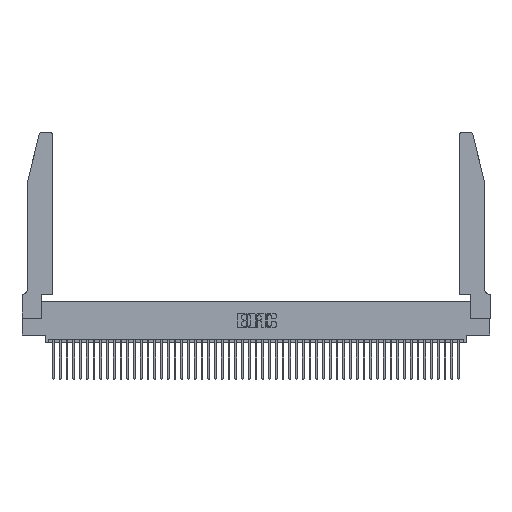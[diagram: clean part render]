
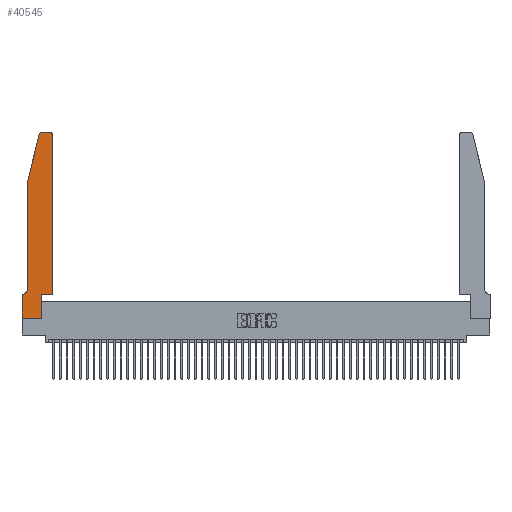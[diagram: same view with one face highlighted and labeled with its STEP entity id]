
A CAD part, top view. The second image highlights one B-rep face of the part: STEP entity #40545.
In plain terms, the highlighted planar face has unit normal (0, 0, 1).
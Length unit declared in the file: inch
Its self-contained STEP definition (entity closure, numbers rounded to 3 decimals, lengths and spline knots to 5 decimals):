
#895 = AXIS2_PLACEMENT_3D ( 'NONE', #5784, #1733, #40382 ) ;
#1687 = ORIENTED_EDGE ( 'NONE', *, *, #38924, .T. ) ;
#1733 = DIRECTION ( 'NONE',  ( 0., 0., 1. ) ) ;
#1961 = AXIS2_PLACEMENT_3D ( 'NONE', #10646, #10140, #18098 ) ;
#3257 = CARTESIAN_POINT ( 'NONE',  ( 0.2605, 2.75, 0.37 ) ) ;
#4375 = ORIENTED_EDGE ( 'NONE', *, *, #48775, .T. ) ;
#4608 = LINE ( 'NONE', #48149, #23422 ) ;
#4831 = EDGE_CURVE ( 'NONE', #44853, #16241, #30279, .T. ) ;
#4845 = ORIENTED_EDGE ( 'NONE', *, *, #49633, .T. ) ;
#5235 = EDGE_CURVE ( 'NONE', #25464, #12131, #12644, .T. ) ;
#5326 = VERTEX_POINT ( 'NONE', #26094 ) ;
#5435 = CARTESIAN_POINT ( 'NONE',  ( 0.4505, 0.35, 0.37 ) ) ;
#5784 = CARTESIAN_POINT ( 'NONE',  ( 0.284, 2.72, 0.37 ) ) ;
#5933 = CARTESIAN_POINT ( 'NONE',  ( 0.0755, 2., 0.37 ) ) ;
#7418 = EDGE_CURVE ( 'NONE', #37153, #15062, #4608, .T. ) ;
#8708 = PLANE ( 'NONE',  #10379 ) ;
#8995 = CARTESIAN_POINT ( 'NONE',  ( 0.2865, 0.35, 0.37 ) ) ;
#9903 = EDGE_CURVE ( 'NONE', #29496, #5326, #27393, .T. ) ;
#10049 = EDGE_CURVE ( 'NONE', #49851, #44853, #29752, .T. ) ;
#10064 = VECTOR ( 'NONE', #48953, 39.37008 ) ;
#10140 = DIRECTION ( 'NONE',  ( 0., 0., -1. ) ) ;
#10379 = AXIS2_PLACEMENT_3D ( 'NONE', #28350, #28513, #24805 ) ;
#10646 = CARTESIAN_POINT ( 'NONE',  ( 0.0055, 0.42, 0.37 ) ) ;
#10934 = CARTESIAN_POINT ( 'NONE',  ( 0.2865, 0., 0.37 ) ) ;
#11265 = CARTESIAN_POINT ( 'NONE',  ( 0.25487, 2.72718, 0.37 ) ) ;
#11903 = DIRECTION ( 'NONE',  ( 0., -1., 0. ) ) ;
#12131 = VERTEX_POINT ( 'NONE', #30305 ) ;
#12159 = DIRECTION ( 'NONE',  ( 0., 0., 1. ) ) ;
#12335 = VERTEX_POINT ( 'NONE', #20091 ) ;
#12644 = LINE ( 'NONE', #22041, #34484 ) ;
#12860 = DIRECTION ( 'NONE',  ( 0., -1., 0. ) ) ;
#15062 = VERTEX_POINT ( 'NONE', #40187 ) ;
#15099 = CARTESIAN_POINT ( 'NONE',  ( 0.4505, 0.35, 0.37 ) ) ;
#15204 = EDGE_CURVE ( 'NONE', #5326, #25464, #15318, .T. ) ;
#15313 = EDGE_CURVE ( 'NONE', #16241, #20858, #47471, .T. ) ;
#15318 = LINE ( 'NONE', #5435, #43827 ) ;
#16241 = VERTEX_POINT ( 'NONE', #36852 ) ;
#16560 = FACE_OUTER_BOUND ( 'NONE', #43629, .T. ) ;
#16762 = LINE ( 'NONE', #29061, #10064 ) ;
#17119 = VECTOR ( 'NONE', #35952, 39.37008 ) ;
#18098 = DIRECTION ( 'NONE',  ( -1., 0., 0. ) ) ;
#18165 = VECTOR ( 'NONE', #26978, 39.37008 ) ;
#20091 = CARTESIAN_POINT ( 'NONE',  ( 0.284, 2.75, 0.37 ) ) ;
#20858 = VERTEX_POINT ( 'NONE', #25593 ) ;
#22041 = CARTESIAN_POINT ( 'NONE',  ( 0.4505, 0.35, 0.37 ) ) ;
#23422 = VECTOR ( 'NONE', #12860, 39.37008 ) ;
#23681 = ORIENTED_EDGE ( 'NONE', *, *, #46556, .T. ) ;
#24133 = CIRCLE ( 'NONE', #895, 0.03 ) ;
#24805 = DIRECTION ( 'NONE',  ( 1., 0., 0. ) ) ;
#25464 = VERTEX_POINT ( 'NONE', #15099 ) ;
#25593 = CARTESIAN_POINT ( 'NONE',  ( 0.0055, 0.35, 0.37 ) ) ;
#25927 = DIRECTION ( 'NONE',  ( 0., 1., 0. ) ) ;
#26094 = CARTESIAN_POINT ( 'NONE',  ( 0.2865, 0.35, 0.37 ) ) ;
#26978 = DIRECTION ( 'NONE',  ( -1., 0., 0. ) ) ;
#27210 = EDGE_CURVE ( 'NONE', #30977, #12335, #43808, .T. ) ;
#27241 = AXIS2_PLACEMENT_3D ( 'NONE', #35045, #12159, #39313 ) ;
#27393 = LINE ( 'NONE', #8995, #17119 ) ;
#28350 = CARTESIAN_POINT ( 'NONE',  ( 0., 0.35, 0.37 ) ) ;
#28431 = VECTOR ( 'NONE', #11903, 39.37008 ) ;
#28513 = DIRECTION ( 'NONE',  ( 0., 0., 1. ) ) ;
#28637 = VECTOR ( 'NONE', #42072, 39.37008 ) ;
#29061 = CARTESIAN_POINT ( 'NONE',  ( 0., 0., 0.37 ) ) ;
#29496 = VERTEX_POINT ( 'NONE', #10934 ) ;
#29752 = LINE ( 'NONE', #32724, #48016 ) ;
#30279 = LINE ( 'NONE', #42800, #28431 ) ;
#30305 = CARTESIAN_POINT ( 'NONE',  ( 0.4505, 2.72, 0.37 ) ) ;
#30977 = VERTEX_POINT ( 'NONE', #37005 ) ;
#31026 = ORIENTED_EDGE ( 'NONE', *, *, #9903, .T. ) ;
#32724 = CARTESIAN_POINT ( 'NONE',  ( 0.0755, 2., 0.37 ) ) ;
#33470 = ORIENTED_EDGE ( 'NONE', *, *, #5235, .T. ) ;
#34265 = ORIENTED_EDGE ( 'NONE', *, *, #15313, .T. ) ;
#34484 = VECTOR ( 'NONE', #25927, 39.37008 ) ;
#34774 = CARTESIAN_POINT ( 'NONE',  ( 0.0755, 0.35, 0.37 ) ) ;
#34918 = CIRCLE ( 'NONE', #27241, 0.03 ) ;
#35045 = CARTESIAN_POINT ( 'NONE',  ( 0.4205, 2.72, 0.37 ) ) ;
#35952 = DIRECTION ( 'NONE',  ( 0., 1., 0. ) ) ;
#36774 = DIRECTION ( 'NONE',  ( -0.239, -0.971, 0. ) ) ;
#36852 = CARTESIAN_POINT ( 'NONE',  ( 0.0755, 0.42, 0.37 ) ) ;
#37005 = CARTESIAN_POINT ( 'NONE',  ( 0.4205, 2.75, 0.37 ) ) ;
#37153 = VERTEX_POINT ( 'NONE', #43700 ) ;
#38924 = EDGE_CURVE ( 'NONE', #12131, #30977, #34918, .T. ) ;
#39313 = DIRECTION ( 'NONE',  ( 1., 0., 0. ) ) ;
#40062 = ORIENTED_EDGE ( 'NONE', *, *, #4831, .T. ) ;
#40187 = CARTESIAN_POINT ( 'NONE',  ( 0., 0., 0.37 ) ) ;
#40353 = DIRECTION ( 'NONE',  ( 1., 0., 0. ) ) ;
#40382 = DIRECTION ( 'NONE',  ( 1., 0., 0. ) ) ;
#40545 = ADVANCED_FACE ( 'NONE', ( #16560 ), #8708, .T. ) ;
#41260 = ORIENTED_EDGE ( 'NONE', *, *, #27210, .T. ) ;
#41437 = ORIENTED_EDGE ( 'NONE', *, *, #10049, .T. ) ;
#42072 = DIRECTION ( 'NONE',  ( -1., 0., 0. ) ) ;
#42800 = CARTESIAN_POINT ( 'NONE',  ( 0.0755, 2., 0.37 ) ) ;
#42961 = ORIENTED_EDGE ( 'NONE', *, *, #7418, .T. ) ;
#43629 = EDGE_LOOP ( 'NONE', ( #41260, #4375, #41437, #40062, #34265, #23681, #42961, #4845, #31026, #48952, #33470, #1687 ) ) ;
#43700 = CARTESIAN_POINT ( 'NONE',  ( 0., 0.35, 0.37 ) ) ;
#43808 = LINE ( 'NONE', #3257, #28637 ) ;
#43827 = VECTOR ( 'NONE', #40353, 39.37008 ) ;
#44853 = VERTEX_POINT ( 'NONE', #5933 ) ;
#46556 = EDGE_CURVE ( 'NONE', #20858, #37153, #47340, .T. ) ;
#47340 = LINE ( 'NONE', #34774, #18165 ) ;
#47471 = CIRCLE ( 'NONE', #1961, 0.07 ) ;
#48016 = VECTOR ( 'NONE', #36774, 39.37008 ) ;
#48149 = CARTESIAN_POINT ( 'NONE',  ( 0., 0., 0.37 ) ) ;
#48775 = EDGE_CURVE ( 'NONE', #12335, #49851, #24133, .T. ) ;
#48952 = ORIENTED_EDGE ( 'NONE', *, *, #15204, .T. ) ;
#48953 = DIRECTION ( 'NONE',  ( 1., 0., 0. ) ) ;
#49633 = EDGE_CURVE ( 'NONE', #15062, #29496, #16762, .T. ) ;
#49851 = VERTEX_POINT ( 'NONE', #11265 ) ;
